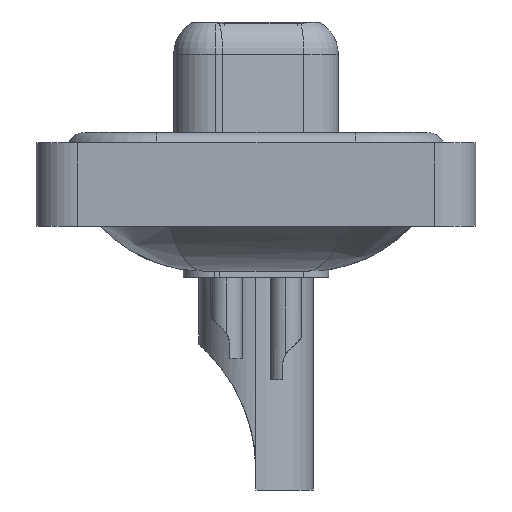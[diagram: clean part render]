
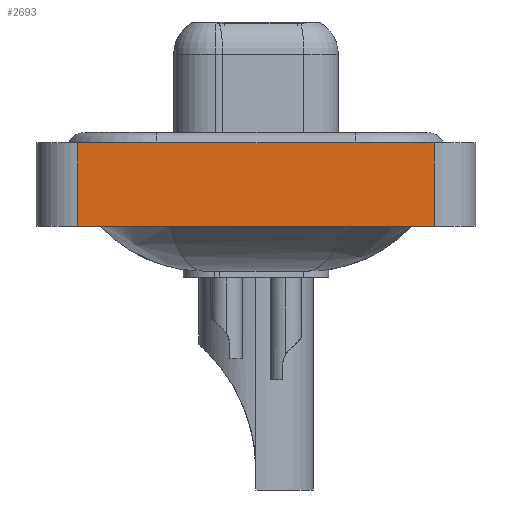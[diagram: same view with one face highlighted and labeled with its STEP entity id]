
A CAD part, left-side view. The second image highlights one B-rep face of the part: STEP entity #2693.
In plain terms, the highlighted planar face has unit normal (-1, 0, 0).
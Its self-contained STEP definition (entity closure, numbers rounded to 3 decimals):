
#678 = EDGE_CURVE ( 'NONE', #4753, #22199, #2529, .T. ) ;
#874 = EDGE_CURVE ( 'NONE', #21758, #4753, #22481, .T. ) ;
#1435 = VECTOR ( 'NONE', #5801, 1000. ) ;
#1462 = DIRECTION ( 'NONE',  ( 0., 0., 1. ) ) ;
#2529 = LINE ( 'NONE', #22036, #11251 ) ;
#2693 = ADVANCED_FACE ( 'NONE', ( #13549 ), #13327, .T. ) ;
#4315 = LINE ( 'NONE', #16099, #1435 ) ;
#4385 = CARTESIAN_POINT ( 'NONE',  ( -7.3, -8.55, -3.6 ) ) ;
#4753 = VERTEX_POINT ( 'NONE', #4385 ) ;
#5544 = EDGE_LOOP ( 'NONE', ( #15440, #19151, #16549, #18795 ) ) ;
#5801 = DIRECTION ( 'NONE',  ( 0., 0., 1. ) ) ;
#6197 = DIRECTION ( 'NONE',  ( 0., 0., 1. ) ) ;
#8093 = CARTESIAN_POINT ( 'NONE',  ( -7.3, -8.55, -3.6 ) ) ;
#8906 = LINE ( 'NONE', #13188, #15713 ) ;
#9438 = CARTESIAN_POINT ( 'NONE',  ( -7.3, -8.55, 0.4 ) ) ;
#10203 = CARTESIAN_POINT ( 'NONE',  ( -7.3, 8.55, 0.4 ) ) ;
#11251 = VECTOR ( 'NONE', #6197, 1000. ) ;
#12766 = CARTESIAN_POINT ( 'NONE',  ( -7.3, 8.55, -3.6 ) ) ;
#13188 = CARTESIAN_POINT ( 'NONE',  ( -7.3, -8.55, 0.4 ) ) ;
#13327 = PLANE ( 'NONE',  #14227 ) ;
#13408 = DIRECTION ( 'NONE',  ( 0., -1., 0. ) ) ;
#13549 = FACE_OUTER_BOUND ( 'NONE', #5544, .T. ) ;
#14074 = VERTEX_POINT ( 'NONE', #10203 ) ;
#14227 = AXIS2_PLACEMENT_3D ( 'NONE', #8093, #16903, #1462 ) ;
#14255 = EDGE_CURVE ( 'NONE', #21758, #14074, #4315, .T. ) ;
#15440 = ORIENTED_EDGE ( 'NONE', *, *, #678, .T. ) ;
#15713 = VECTOR ( 'NONE', #13408, 1000. ) ;
#16099 = CARTESIAN_POINT ( 'NONE',  ( -7.3, 8.55, -3.6 ) ) ;
#16549 = ORIENTED_EDGE ( 'NONE', *, *, #14255, .F. ) ;
#16903 = DIRECTION ( 'NONE',  ( -1., 0., 0. ) ) ;
#17841 = VECTOR ( 'NONE', #20741, 1000. ) ;
#18520 = EDGE_CURVE ( 'NONE', #14074, #22199, #8906, .T. ) ;
#18795 = ORIENTED_EDGE ( 'NONE', *, *, #874, .T. ) ;
#19151 = ORIENTED_EDGE ( 'NONE', *, *, #18520, .F. ) ;
#20741 = DIRECTION ( 'NONE',  ( 0., -1., 0. ) ) ;
#21758 = VERTEX_POINT ( 'NONE', #12766 ) ;
#22036 = CARTESIAN_POINT ( 'NONE',  ( -7.3, -8.55, -3.6 ) ) ;
#22199 = VERTEX_POINT ( 'NONE', #9438 ) ;
#22481 = LINE ( 'NONE', #22579, #17841 ) ;
#22579 = CARTESIAN_POINT ( 'NONE',  ( -7.3, -8.55, -3.6 ) ) ;
